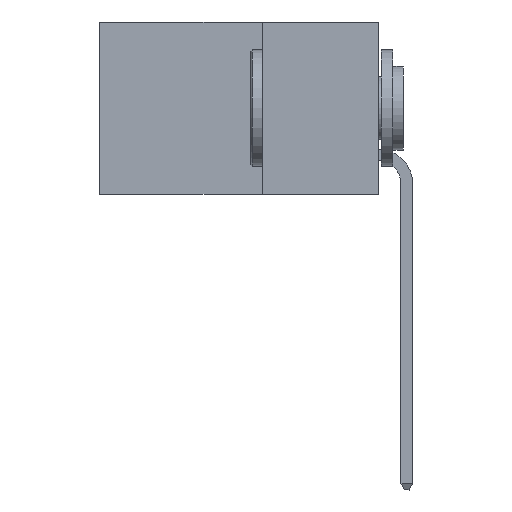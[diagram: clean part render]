
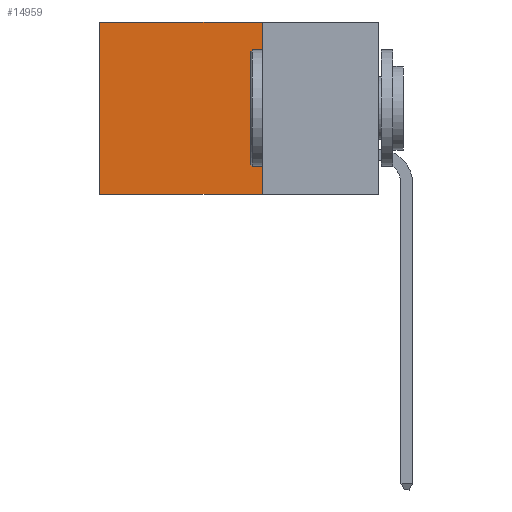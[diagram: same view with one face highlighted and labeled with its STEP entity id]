
A CAD part, left-side view. The second image highlights one B-rep face of the part: STEP entity #14959.
In plain terms, the highlighted planar face has unit normal (-1, 0, 0).
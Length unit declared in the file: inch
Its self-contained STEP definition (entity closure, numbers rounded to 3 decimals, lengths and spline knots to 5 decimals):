
#618 = CARTESIAN_POINT ( 'NONE',  ( 0.2615, 0.6, 0. ) ) ;
#1731 = LINE ( 'NONE', #3533, #15179 ) ;
#1760 = VECTOR ( 'NONE', #7854, 39.37008 ) ;
#3100 = FACE_OUTER_BOUND ( 'NONE', #21581, .T. ) ;
#3260 = CARTESIAN_POINT ( 'NONE',  ( 0.2615, 0.6, -0.37 ) ) ;
#3533 = CARTESIAN_POINT ( 'NONE',  ( 0.2615, 0.25, 0. ) ) ;
#4295 = CARTESIAN_POINT ( 'NONE',  ( 0.2615, 0.25, -0.37 ) ) ;
#4597 = VERTEX_POINT ( 'NONE', #10830 ) ;
#5080 = LINE ( 'NONE', #20411, #14201 ) ;
#6071 = EDGE_CURVE ( 'NONE', #15716, #10335, #15288, .T. ) ;
#6335 = DIRECTION ( 'NONE',  ( 0., 0., -1. ) ) ;
#6337 = EDGE_CURVE ( 'NONE', #9427, #4597, #5080, .T. ) ;
#6394 = ORIENTED_EDGE ( 'NONE', *, *, #11532, .F. ) ;
#6399 = AXIS2_PLACEMENT_3D ( 'NONE', #16636, #9469, #6335 ) ;
#6727 = ORIENTED_EDGE ( 'NONE', *, *, #19587, .T. ) ;
#7854 = DIRECTION ( 'NONE',  ( 0., 1., 0. ) ) ;
#8319 = DIRECTION ( 'NONE',  ( 0., 0., -1. ) ) ;
#9427 = VERTEX_POINT ( 'NONE', #21046 ) ;
#9469 = DIRECTION ( 'NONE',  ( 1., 0., 0. ) ) ;
#10335 = VERTEX_POINT ( 'NONE', #3260 ) ;
#10830 = CARTESIAN_POINT ( 'NONE',  ( 0.2615, 0.25, -0.37 ) ) ;
#11532 = EDGE_CURVE ( 'NONE', #4597, #10335, #18254, .T. ) ;
#11588 = CARTESIAN_POINT ( 'NONE',  ( 0.2615, 0.6, -0.37 ) ) ;
#12369 = DIRECTION ( 'NONE',  ( 0., 1., 0. ) ) ;
#14201 = VECTOR ( 'NONE', #8319, 39.37008 ) ;
#14896 = ORIENTED_EDGE ( 'NONE', *, *, #6337, .F. ) ;
#14959 = ADVANCED_FACE ( 'NONE', ( #3100 ), #21584, .F. ) ;
#15179 = VECTOR ( 'NONE', #12369, 39.37008 ) ;
#15288 = LINE ( 'NONE', #11588, #17763 ) ;
#15716 = VERTEX_POINT ( 'NONE', #618 ) ;
#16636 = CARTESIAN_POINT ( 'NONE',  ( 0.2615, 0.25, -0.37 ) ) ;
#16854 = DIRECTION ( 'NONE',  ( 0., 0., -1. ) ) ;
#17763 = VECTOR ( 'NONE', #16854, 39.37008 ) ;
#18254 = LINE ( 'NONE', #4295, #1760 ) ;
#19587 = EDGE_CURVE ( 'NONE', #9427, #15716, #1731, .T. ) ;
#20411 = CARTESIAN_POINT ( 'NONE',  ( 0.2615, 0.25, -0.37 ) ) ;
#21046 = CARTESIAN_POINT ( 'NONE',  ( 0.2615, 0.25, 0. ) ) ;
#21301 = ORIENTED_EDGE ( 'NONE', *, *, #6071, .T. ) ;
#21581 = EDGE_LOOP ( 'NONE', ( #21301, #6394, #14896, #6727 ) ) ;
#21584 = PLANE ( 'NONE',  #6399 ) ;
